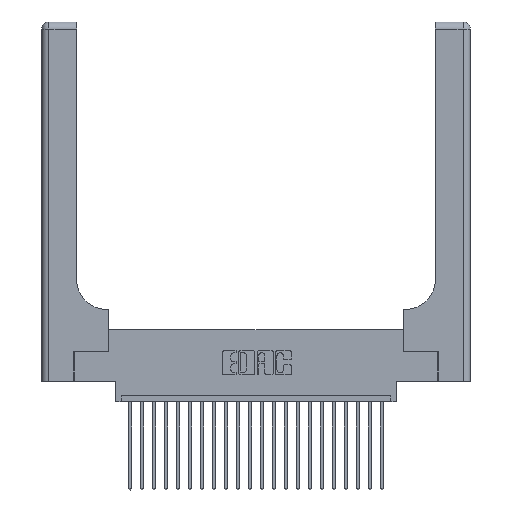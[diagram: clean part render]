
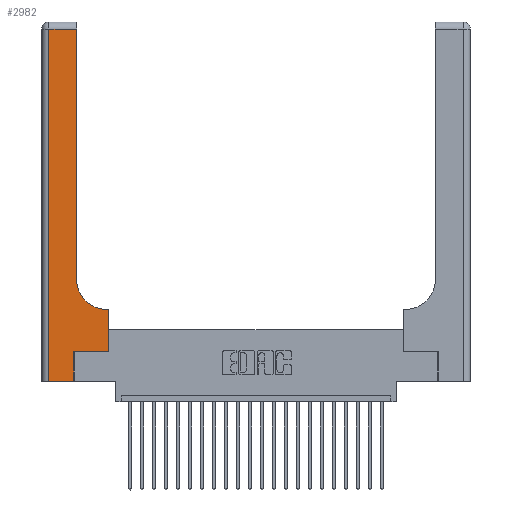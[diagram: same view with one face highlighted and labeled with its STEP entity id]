
A CAD part, top view. The second image highlights one B-rep face of the part: STEP entity #2982.
In plain terms, the highlighted planar face has unit normal (0, 0, 1).
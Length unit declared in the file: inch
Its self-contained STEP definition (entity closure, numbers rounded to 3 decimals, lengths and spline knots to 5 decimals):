
#282 = AXIS2_PLACEMENT_3D ( 'NONE', #2936, #23657, #4802 ) ;
#407 = VERTEX_POINT ( 'NONE', #9194 ) ;
#431 = AXIS2_PLACEMENT_3D ( 'NONE', #19029, #21282, #2011 ) ;
#758 = CARTESIAN_POINT ( 'NONE',  ( 0.5585, 0.6, 0.37 ) ) ;
#1084 = DIRECTION ( 'NONE',  ( 0., 1., 0. ) ) ;
#1114 = PLANE ( 'NONE',  #282 ) ;
#1792 = VERTEX_POINT ( 'NONE', #21187 ) ;
#2011 = DIRECTION ( 'NONE',  ( 1., 0., 0. ) ) ;
#2366 = EDGE_LOOP ( 'NONE', ( #20485, #5989, #5796, #8196, #24306, #16465, #18100, #6919, #3939 ) ) ;
#2371 = CARTESIAN_POINT ( 'NONE',  ( 0.5415, 0.6, 0.37 ) ) ;
#2936 = CARTESIAN_POINT ( 'NONE',  ( 0., 3., 0.37 ) ) ;
#2982 = ADVANCED_FACE ( 'NONE', ( #19171 ), #1114, .F. ) ;
#3939 = ORIENTED_EDGE ( 'NONE', *, *, #13412, .T. ) ;
#4186 = CARTESIAN_POINT ( 'NONE',  ( 0.269, 0.25, 0.37 ) ) ;
#4641 = LINE ( 'NONE', #6600, #24557 ) ;
#4802 = DIRECTION ( 'NONE',  ( -1., 0., 0. ) ) ;
#4847 = VECTOR ( 'NONE', #24373, 39.37008 ) ;
#5108 = DIRECTION ( 'NONE',  ( 1., 0., 0. ) ) ;
#5228 = EDGE_CURVE ( 'NONE', #17929, #14113, #23835, .T. ) ;
#5796 = ORIENTED_EDGE ( 'NONE', *, *, #7826, .T. ) ;
#5989 = ORIENTED_EDGE ( 'NONE', *, *, #15648, .T. ) ;
#6600 = CARTESIAN_POINT ( 'NONE',  ( 0.2915, 3., 0.37 ) ) ;
#6919 = ORIENTED_EDGE ( 'NONE', *, *, #16438, .T. ) ;
#7155 = CARTESIAN_POINT ( 'NONE',  ( 0., 2.94, 0.37 ) ) ;
#7826 = EDGE_CURVE ( 'NONE', #21721, #1792, #17788, .T. ) ;
#7889 = VERTEX_POINT ( 'NONE', #15551 ) ;
#8196 = ORIENTED_EDGE ( 'NONE', *, *, #19136, .T. ) ;
#8306 = CARTESIAN_POINT ( 'NONE',  ( 0.5585, 0.25, 0.37 ) ) ;
#8851 = LINE ( 'NONE', #4186, #21963 ) ;
#8918 = DIRECTION ( 'NONE',  ( 0., -1., 0. ) ) ;
#8934 = EDGE_CURVE ( 'NONE', #7889, #18113, #4641, .T. ) ;
#9194 = CARTESIAN_POINT ( 'NONE',  ( 0.269, 0., 0.37 ) ) ;
#9659 = CIRCLE ( 'NONE', #431, 0.25 ) ;
#9960 = LINE ( 'NONE', #10832, #24552 ) ;
#10832 = CARTESIAN_POINT ( 'NONE',  ( 0., 0., 0.37 ) ) ;
#11988 = VERTEX_POINT ( 'NONE', #17211 ) ;
#12533 = CARTESIAN_POINT ( 'NONE',  ( 0.06, 3., 0.37 ) ) ;
#13412 = EDGE_CURVE ( 'NONE', #14606, #7889, #9659, .T. ) ;
#13715 = VECTOR ( 'NONE', #1084, 39.37008 ) ;
#14113 = VERTEX_POINT ( 'NONE', #758 ) ;
#14199 = DIRECTION ( 'NONE',  ( 0., 1., 0. ) ) ;
#14606 = VERTEX_POINT ( 'NONE', #2371 ) ;
#15551 = CARTESIAN_POINT ( 'NONE',  ( 0.2915, 0.85, 0.37 ) ) ;
#15622 = CARTESIAN_POINT ( 'NONE',  ( 0.5585, 0.25, 0.37 ) ) ;
#15648 = EDGE_CURVE ( 'NONE', #18113, #21721, #16436, .T. ) ;
#16178 = DIRECTION ( 'NONE',  ( 0., 1., 0. ) ) ;
#16436 = LINE ( 'NONE', #7155, #4847 ) ;
#16438 = EDGE_CURVE ( 'NONE', #14113, #14606, #20294, .T. ) ;
#16465 = ORIENTED_EDGE ( 'NONE', *, *, #17842, .T. ) ;
#16764 = CARTESIAN_POINT ( 'NONE',  ( 0.2915, 2.94, 0.37 ) ) ;
#17211 = CARTESIAN_POINT ( 'NONE',  ( 0.269, 0.25, 0.37 ) ) ;
#17478 = DIRECTION ( 'NONE',  ( 1., 0., 0. ) ) ;
#17788 = LINE ( 'NONE', #12533, #23140 ) ;
#17842 = EDGE_CURVE ( 'NONE', #11988, #17929, #8851, .T. ) ;
#17929 = VERTEX_POINT ( 'NONE', #15622 ) ;
#18100 = ORIENTED_EDGE ( 'NONE', *, *, #5228, .T. ) ;
#18104 = CARTESIAN_POINT ( 'NONE',  ( 0.269, 0., 0.37 ) ) ;
#18113 = VERTEX_POINT ( 'NONE', #16764 ) ;
#18949 = DIRECTION ( 'NONE',  ( -1., 0., 0. ) ) ;
#19029 = CARTESIAN_POINT ( 'NONE',  ( 0.5415, 0.85, 0.37 ) ) ;
#19136 = EDGE_CURVE ( 'NONE', #1792, #407, #9960, .T. ) ;
#19149 = VECTOR ( 'NONE', #16178, 39.37008 ) ;
#19171 = FACE_OUTER_BOUND ( 'NONE', #2366, .T. ) ;
#19620 = CARTESIAN_POINT ( 'NONE',  ( 0.06, 2.94, 0.37 ) ) ;
#20294 = LINE ( 'NONE', #22689, #22937 ) ;
#20485 = ORIENTED_EDGE ( 'NONE', *, *, #8934, .T. ) ;
#20755 = EDGE_CURVE ( 'NONE', #407, #11988, #22140, .T. ) ;
#21187 = CARTESIAN_POINT ( 'NONE',  ( 0.06, 0., 0.37 ) ) ;
#21282 = DIRECTION ( 'NONE',  ( 0., 0., -1. ) ) ;
#21721 = VERTEX_POINT ( 'NONE', #19620 ) ;
#21963 = VECTOR ( 'NONE', #17478, 39.37008 ) ;
#22140 = LINE ( 'NONE', #18104, #19149 ) ;
#22689 = CARTESIAN_POINT ( 'NONE',  ( 0.2915, 0.6, 0.37 ) ) ;
#22937 = VECTOR ( 'NONE', #18949, 39.37008 ) ;
#23140 = VECTOR ( 'NONE', #8918, 39.37008 ) ;
#23657 = DIRECTION ( 'NONE',  ( 0., 0., -1. ) ) ;
#23835 = LINE ( 'NONE', #8306, #13715 ) ;
#24306 = ORIENTED_EDGE ( 'NONE', *, *, #20755, .T. ) ;
#24373 = DIRECTION ( 'NONE',  ( -1., 0., 0. ) ) ;
#24552 = VECTOR ( 'NONE', #5108, 39.37008 ) ;
#24557 = VECTOR ( 'NONE', #14199, 39.37008 ) ;
